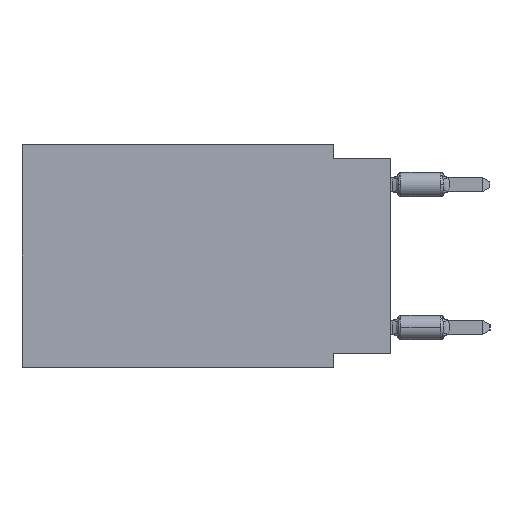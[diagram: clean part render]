
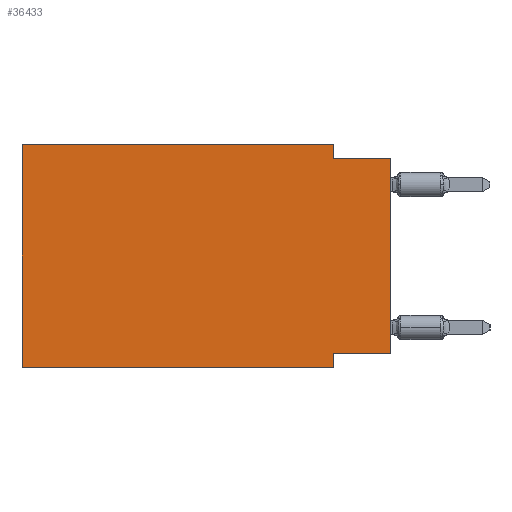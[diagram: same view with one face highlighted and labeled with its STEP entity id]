
A CAD part, left-side view. The second image highlights one B-rep face of the part: STEP entity #36433.
In plain terms, the highlighted planar face has unit normal (-1, 0, 0).
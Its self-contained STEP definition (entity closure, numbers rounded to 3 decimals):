
#104 = EDGE_CURVE ( 'NONE', #4736, #24918, #30107, .T. ) ;
#201 = VECTOR ( 'NONE', #17437, 1000. ) ;
#820 = DIRECTION ( 'NONE',  ( 0., 0., -1. ) ) ;
#919 = CARTESIAN_POINT ( 'NONE',  ( 0., 2.54, -9.906 ) ) ;
#2254 = VERTEX_POINT ( 'NONE', #9261 ) ;
#3130 = CARTESIAN_POINT ( 'NONE',  ( 0., 16.383, 0. ) ) ;
#3250 = CARTESIAN_POINT ( 'NONE',  ( 0., 0., -0.635 ) ) ;
#4736 = VERTEX_POINT ( 'NONE', #13095 ) ;
#4838 = FACE_OUTER_BOUND ( 'NONE', #10657, .T. ) ;
#5826 = EDGE_CURVE ( 'NONE', #22954, #25812, #41591, .T. ) ;
#6469 = ORIENTED_EDGE ( 'NONE', *, *, #26259, .F. ) ;
#7339 = ORIENTED_EDGE ( 'NONE', *, *, #35817, .F. ) ;
#7915 = DIRECTION ( 'NONE',  ( 1., 0., 0. ) ) ;
#8571 = DIRECTION ( 'NONE',  ( 0., -1., 0. ) ) ;
#8862 = CARTESIAN_POINT ( 'NONE',  ( 0., 0., 0. ) ) ;
#9261 = CARTESIAN_POINT ( 'NONE',  ( 0., 2.54, -9.271 ) ) ;
#10226 = VERTEX_POINT ( 'NONE', #27906 ) ;
#10657 = EDGE_LOOP ( 'NONE', ( #36838, #31938, #38477, #26153, #6469, #26989, #42929, #7339 ) ) ;
#13095 = CARTESIAN_POINT ( 'NONE',  ( 0., 16.383, 0. ) ) ;
#14726 = LINE ( 'NONE', #15167, #43004 ) ;
#15167 = CARTESIAN_POINT ( 'NONE',  ( 0., 16.383, -9.906 ) ) ;
#15823 = EDGE_CURVE ( 'NONE', #24918, #29706, #30376, .T. ) ;
#17437 = DIRECTION ( 'NONE',  ( 0., -1., 0. ) ) ;
#17877 = DIRECTION ( 'NONE',  ( 0., 1., 0. ) ) ;
#18824 = DIRECTION ( 'NONE',  ( 0., 0., -1. ) ) ;
#19740 = EDGE_CURVE ( 'NONE', #2254, #35121, #32963, .T. ) ;
#22931 = CARTESIAN_POINT ( 'NONE',  ( 0., 2.54, 0. ) ) ;
#22954 = VERTEX_POINT ( 'NONE', #24436 ) ;
#24338 = LINE ( 'NONE', #3130, #30962 ) ;
#24436 = CARTESIAN_POINT ( 'NONE',  ( 0., 0., -9.271 ) ) ;
#24578 = DIRECTION ( 'NONE',  ( 0., 0., 1. ) ) ;
#24918 = VERTEX_POINT ( 'NONE', #22931 ) ;
#25812 = VERTEX_POINT ( 'NONE', #3250 ) ;
#26153 = ORIENTED_EDGE ( 'NONE', *, *, #104, .F. ) ;
#26259 = EDGE_CURVE ( 'NONE', #10226, #4736, #24338, .T. ) ;
#26989 = ORIENTED_EDGE ( 'NONE', *, *, #34483, .T. ) ;
#27906 = CARTESIAN_POINT ( 'NONE',  ( 0., 16.383, -9.906 ) ) ;
#27935 = EDGE_CURVE ( 'NONE', #29706, #25812, #28720, .T. ) ;
#28720 = LINE ( 'NONE', #32258, #201 ) ;
#29173 = LINE ( 'NONE', #32224, #46154 ) ;
#29611 = CARTESIAN_POINT ( 'NONE',  ( 0., 2.54, -0.635 ) ) ;
#29706 = VERTEX_POINT ( 'NONE', #29611 ) ;
#30107 = LINE ( 'NONE', #44488, #32816 ) ;
#30376 = LINE ( 'NONE', #37448, #38795 ) ;
#30962 = VECTOR ( 'NONE', #24578, 1000. ) ;
#31104 = AXIS2_PLACEMENT_3D ( 'NONE', #37354, #7915, #820 ) ;
#31335 = DIRECTION ( 'NONE',  ( 0., 0., -1. ) ) ;
#31938 = ORIENTED_EDGE ( 'NONE', *, *, #27935, .F. ) ;
#31970 = VECTOR ( 'NONE', #37355, 1000. ) ;
#32224 = CARTESIAN_POINT ( 'NONE',  ( 0., 0., -9.271 ) ) ;
#32258 = CARTESIAN_POINT ( 'NONE',  ( 0., 0., -0.635 ) ) ;
#32816 = VECTOR ( 'NONE', #41435, 1000. ) ;
#32963 = LINE ( 'NONE', #919, #41310 ) ;
#34483 = EDGE_CURVE ( 'NONE', #10226, #35121, #14726, .T. ) ;
#35121 = VERTEX_POINT ( 'NONE', #38202 ) ;
#35817 = EDGE_CURVE ( 'NONE', #22954, #2254, #29173, .T. ) ;
#36433 = ADVANCED_FACE ( 'NONE', ( #4838 ), #40871, .F. ) ;
#36838 = ORIENTED_EDGE ( 'NONE', *, *, #5826, .T. ) ;
#37354 = CARTESIAN_POINT ( 'NONE',  ( 0., 16.383, 0. ) ) ;
#37355 = DIRECTION ( 'NONE',  ( 0., 0., 1. ) ) ;
#37448 = CARTESIAN_POINT ( 'NONE',  ( 0., 2.54, 0. ) ) ;
#38202 = CARTESIAN_POINT ( 'NONE',  ( 0., 2.54, -9.906 ) ) ;
#38477 = ORIENTED_EDGE ( 'NONE', *, *, #15823, .F. ) ;
#38795 = VECTOR ( 'NONE', #31335, 1000. ) ;
#40871 = PLANE ( 'NONE',  #31104 ) ;
#41310 = VECTOR ( 'NONE', #18824, 1000. ) ;
#41435 = DIRECTION ( 'NONE',  ( 0., -1., 0. ) ) ;
#41591 = LINE ( 'NONE', #8862, #31970 ) ;
#42929 = ORIENTED_EDGE ( 'NONE', *, *, #19740, .F. ) ;
#43004 = VECTOR ( 'NONE', #8571, 1000. ) ;
#44488 = CARTESIAN_POINT ( 'NONE',  ( 0., 16.383, 0. ) ) ;
#46154 = VECTOR ( 'NONE', #17877, 1000. ) ;
